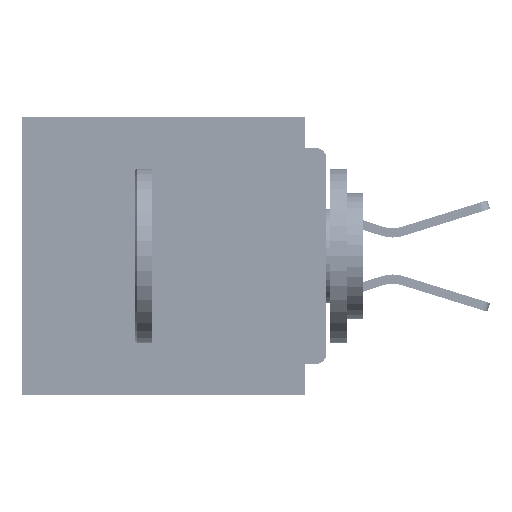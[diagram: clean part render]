
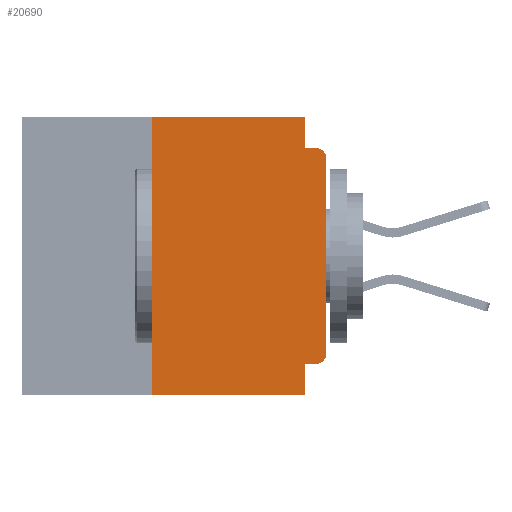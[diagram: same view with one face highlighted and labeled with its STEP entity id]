
A CAD part, left-side view. The second image highlights one B-rep face of the part: STEP entity #20690.
In plain terms, the highlighted planar face has unit normal (-1, 0, 0).
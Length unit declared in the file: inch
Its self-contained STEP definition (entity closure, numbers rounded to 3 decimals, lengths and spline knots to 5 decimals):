
#44 = EDGE_CURVE ( 'NONE', #27353, #6073, #63525, .T. ) ;
#501 = VERTEX_POINT ( 'NONE', #14416 ) ;
#1421 = VECTOR ( 'NONE', #57677, 39.37008 ) ;
#1574 = DIRECTION ( 'NONE',  ( 1., 0., 0. ) ) ;
#3432 = VERTEX_POINT ( 'NONE', #3562 ) ;
#3562 = CARTESIAN_POINT ( 'NONE',  ( 0., 0.031, -0.4 ) ) ;
#3633 = CARTESIAN_POINT ( 'NONE',  ( 0., 0.25, -0.4 ) ) ;
#3945 = LINE ( 'NONE', #61781, #45698 ) ;
#4857 = VECTOR ( 'NONE', #59683, 39.37008 ) ;
#5449 = ORIENTED_EDGE ( 'NONE', *, *, #45376, .F. ) ;
#6073 = VERTEX_POINT ( 'NONE', #26928 ) ;
#6977 = EDGE_CURVE ( 'NONE', #35842, #50853, #59306, .T. ) ;
#7610 = DIRECTION ( 'NONE',  ( 0., -1., 0. ) ) ;
#8024 = EDGE_CURVE ( 'NONE', #501, #3432, #20136, .T. ) ;
#8648 = LINE ( 'NONE', #40757, #34289 ) ;
#11392 = CARTESIAN_POINT ( 'NONE',  ( 0., 0.25, 0. ) ) ;
#11661 = EDGE_CURVE ( 'NONE', #50011, #27353, #28976, .T. ) ;
#12120 = DIRECTION ( 'NONE',  ( 0., 0., -1. ) ) ;
#12932 = VERTEX_POINT ( 'NONE', #3633 ) ;
#14283 = DIRECTION ( 'NONE',  ( 0., 0., 1. ) ) ;
#14416 = CARTESIAN_POINT ( 'NONE',  ( 0., 0.031, -0.355 ) ) ;
#14469 = CARTESIAN_POINT ( 'NONE',  ( 0., 0.031, 0. ) ) ;
#15291 = ORIENTED_EDGE ( 'NONE', *, *, #44, .T. ) ;
#16281 = VECTOR ( 'NONE', #54691, 39.37008 ) ;
#16967 = CARTESIAN_POINT ( 'NONE',  ( 0., 0.015, -0.34 ) ) ;
#20136 = LINE ( 'NONE', #39347, #47290 ) ;
#20208 = EDGE_LOOP ( 'NONE', ( #42064, #15291, #21267, #37463, #30589, #64273, #46294, #54653, #5449, #30256 ) ) ;
#20690 = ADVANCED_FACE ( 'NONE', ( #35740 ), #61273, .F. ) ;
#21267 = ORIENTED_EDGE ( 'NONE', *, *, #37215, .F. ) ;
#22516 = DIRECTION ( 'NONE',  ( 0., 0., -1. ) ) ;
#23877 = AXIS2_PLACEMENT_3D ( 'NONE', #16967, #54957, #22516 ) ;
#24798 = EDGE_CURVE ( 'NONE', #12932, #3432, #38790, .T. ) ;
#26131 = VERTEX_POINT ( 'NONE', #54661 ) ;
#26901 = EDGE_CURVE ( 'NONE', #12932, #55645, #59616, .T. ) ;
#26928 = CARTESIAN_POINT ( 'NONE',  ( 0., 0.015, -0.045 ) ) ;
#27353 = VERTEX_POINT ( 'NONE', #58408 ) ;
#28976 = LINE ( 'NONE', #52350, #68658 ) ;
#30256 = ORIENTED_EDGE ( 'NONE', *, *, #51105, .T. ) ;
#30589 = ORIENTED_EDGE ( 'NONE', *, *, #56005, .F. ) ;
#30724 = CARTESIAN_POINT ( 'NONE',  ( 0., 0.031, 0. ) ) ;
#34289 = VECTOR ( 'NONE', #45935, 39.37008 ) ;
#35522 = AXIS2_PLACEMENT_3D ( 'NONE', #44981, #1574, #39771 ) ;
#35740 = FACE_OUTER_BOUND ( 'NONE', #20208, .T. ) ;
#35842 = VERTEX_POINT ( 'NONE', #14469 ) ;
#37215 = EDGE_CURVE ( 'NONE', #50853, #6073, #64345, .T. ) ;
#37463 = ORIENTED_EDGE ( 'NONE', *, *, #6977, .F. ) ;
#38790 = LINE ( 'NONE', #47256, #65793 ) ;
#39347 = CARTESIAN_POINT ( 'NONE',  ( 0., 0.031, -0.4 ) ) ;
#39771 = DIRECTION ( 'NONE',  ( 0., 0., -1. ) ) ;
#40757 = CARTESIAN_POINT ( 'NONE',  ( 0., 0., -0.355 ) ) ;
#42064 = ORIENTED_EDGE ( 'NONE', *, *, #11661, .T. ) ;
#42726 = DIRECTION ( 'NONE',  ( 0., 0., -1. ) ) ;
#43829 = DIRECTION ( 'NONE',  ( -1., 0., 0. ) ) ;
#44981 = CARTESIAN_POINT ( 'NONE',  ( 0., 0.437, 0. ) ) ;
#45376 = EDGE_CURVE ( 'NONE', #26131, #501, #8648, .T. ) ;
#45698 = VECTOR ( 'NONE', #7610, 39.37008 ) ;
#45935 = DIRECTION ( 'NONE',  ( 0., 1., 0. ) ) ;
#46212 = CARTESIAN_POINT ( 'NONE',  ( 0., 0.015, -0.06 ) ) ;
#46294 = ORIENTED_EDGE ( 'NONE', *, *, #24798, .T. ) ;
#47256 = CARTESIAN_POINT ( 'NONE',  ( 0., 0.437, -0.4 ) ) ;
#47290 = VECTOR ( 'NONE', #12120, 39.37008 ) ;
#48796 = CARTESIAN_POINT ( 'NONE',  ( 0., 0., -0.045 ) ) ;
#50011 = VERTEX_POINT ( 'NONE', #59744 ) ;
#50853 = VERTEX_POINT ( 'NONE', #63015 ) ;
#51105 = EDGE_CURVE ( 'NONE', #26131, #50011, #64813, .T. ) ;
#52350 = CARTESIAN_POINT ( 'NONE',  ( 0., 0., 0. ) ) ;
#52714 = DIRECTION ( 'NONE',  ( 0., -1., 0. ) ) ;
#54642 = AXIS2_PLACEMENT_3D ( 'NONE', #46212, #43829, #42726 ) ;
#54653 = ORIENTED_EDGE ( 'NONE', *, *, #8024, .F. ) ;
#54661 = CARTESIAN_POINT ( 'NONE',  ( 0., 0.015, -0.355 ) ) ;
#54691 = DIRECTION ( 'NONE',  ( 0., 0., 1. ) ) ;
#54957 = DIRECTION ( 'NONE',  ( -1., 0., 0. ) ) ;
#55645 = VERTEX_POINT ( 'NONE', #11392 ) ;
#56005 = EDGE_CURVE ( 'NONE', #55645, #35842, #3945, .T. ) ;
#57677 = DIRECTION ( 'NONE',  ( 0., 0., -1. ) ) ;
#58408 = CARTESIAN_POINT ( 'NONE',  ( 0., 0., -0.06 ) ) ;
#59306 = LINE ( 'NONE', #30724, #1421 ) ;
#59616 = LINE ( 'NONE', #60131, #16281 ) ;
#59683 = DIRECTION ( 'NONE',  ( 0., -1., 0. ) ) ;
#59744 = CARTESIAN_POINT ( 'NONE',  ( 0., 0., -0.34 ) ) ;
#60131 = CARTESIAN_POINT ( 'NONE',  ( 0., 0.25, -0.4 ) ) ;
#61273 = PLANE ( 'NONE',  #35522 ) ;
#61781 = CARTESIAN_POINT ( 'NONE',  ( 0., 0.437, 0. ) ) ;
#63015 = CARTESIAN_POINT ( 'NONE',  ( 0., 0.031, -0.045 ) ) ;
#63525 = CIRCLE ( 'NONE', #54642, 0.015 ) ;
#64273 = ORIENTED_EDGE ( 'NONE', *, *, #26901, .F. ) ;
#64345 = LINE ( 'NONE', #48796, #4857 ) ;
#64813 = CIRCLE ( 'NONE', #23877, 0.015 ) ;
#65793 = VECTOR ( 'NONE', #52714, 39.37008 ) ;
#68658 = VECTOR ( 'NONE', #14283, 39.37008 ) ;
